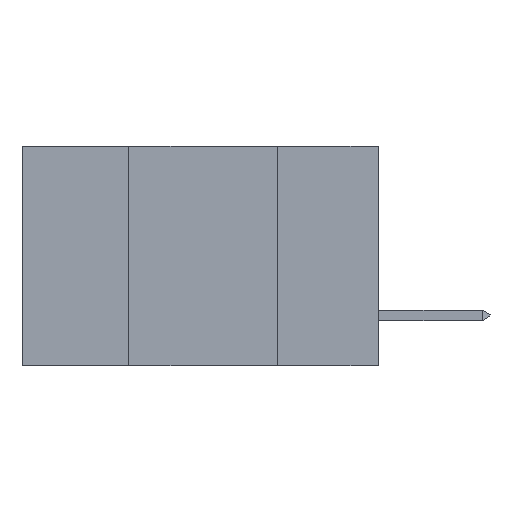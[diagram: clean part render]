
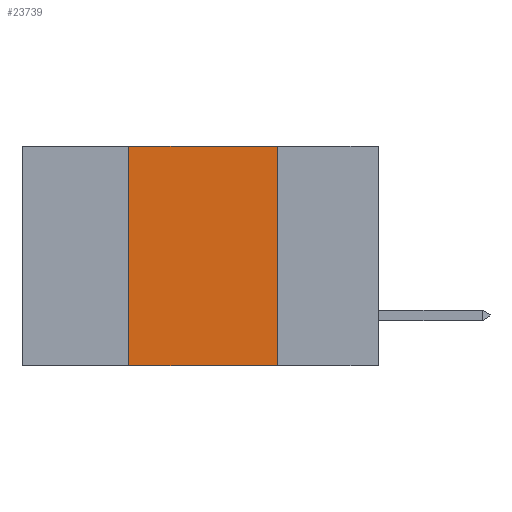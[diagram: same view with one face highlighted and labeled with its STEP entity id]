
A CAD part, left-side view. The second image highlights one B-rep face of the part: STEP entity #23739.
In plain terms, the highlighted planar face has unit normal (-1, 0, 0).
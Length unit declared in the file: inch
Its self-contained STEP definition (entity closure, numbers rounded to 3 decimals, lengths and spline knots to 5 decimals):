
#578 = VERTEX_POINT ( 'NONE', #14400 ) ;
#1663 = VERTEX_POINT ( 'NONE', #5043 ) ;
#1740 = LINE ( 'NONE', #17953, #16033 ) ;
#1945 = CARTESIAN_POINT ( 'NONE',  ( 0., 0.17, -0.37 ) ) ;
#2069 = CARTESIAN_POINT ( 'NONE',  ( 0., 0.6, 0. ) ) ;
#2489 = PLANE ( 'NONE',  #9022 ) ;
#2775 = CARTESIAN_POINT ( 'NONE',  ( 0., 0.17, 0. ) ) ;
#3813 = EDGE_CURVE ( 'NONE', #1663, #17884, #1740, .T. ) ;
#4269 = DIRECTION ( 'NONE',  ( 1., 0., 0. ) ) ;
#4556 = DIRECTION ( 'NONE',  ( 0., 0., -1. ) ) ;
#5043 = CARTESIAN_POINT ( 'NONE',  ( 0., 0.42, 0. ) ) ;
#5257 = LINE ( 'NONE', #8693, #20421 ) ;
#7491 = VECTOR ( 'NONE', #14513, 39.37008 ) ;
#8693 = CARTESIAN_POINT ( 'NONE',  ( 0., 0.42, 0. ) ) ;
#8917 = LINE ( 'NONE', #17741, #9829 ) ;
#8945 = DIRECTION ( 'NONE',  ( 0., 0., 1. ) ) ;
#9022 = AXIS2_PLACEMENT_3D ( 'NONE', #2069, #4269, #9516 ) ;
#9349 = EDGE_CURVE ( 'NONE', #578, #1663, #5257, .T. ) ;
#9516 = DIRECTION ( 'NONE',  ( 0., 0., -1. ) ) ;
#9829 = VECTOR ( 'NONE', #4556, 39.37008 ) ;
#10292 = ORIENTED_EDGE ( 'NONE', *, *, #3813, .F. ) ;
#11657 = EDGE_LOOP ( 'NONE', ( #18509, #10292, #17212, #16828 ) ) ;
#12730 = EDGE_CURVE ( 'NONE', #578, #19247, #23510, .T. ) ;
#13642 = FACE_OUTER_BOUND ( 'NONE', #11657, .T. ) ;
#14400 = CARTESIAN_POINT ( 'NONE',  ( 0., 0.42, -0.37 ) ) ;
#14422 = EDGE_CURVE ( 'NONE', #17884, #19247, #8917, .T. ) ;
#14513 = DIRECTION ( 'NONE',  ( 0., -1., 0. ) ) ;
#16033 = VECTOR ( 'NONE', #16200, 39.37008 ) ;
#16200 = DIRECTION ( 'NONE',  ( 0., -1., 0. ) ) ;
#16828 = ORIENTED_EDGE ( 'NONE', *, *, #12730, .T. ) ;
#17212 = ORIENTED_EDGE ( 'NONE', *, *, #9349, .F. ) ;
#17741 = CARTESIAN_POINT ( 'NONE',  ( 0., 0.17, 0. ) ) ;
#17884 = VERTEX_POINT ( 'NONE', #2775 ) ;
#17953 = CARTESIAN_POINT ( 'NONE',  ( 0., 0.6, 0. ) ) ;
#18509 = ORIENTED_EDGE ( 'NONE', *, *, #14422, .F. ) ;
#19247 = VERTEX_POINT ( 'NONE', #1945 ) ;
#20020 = CARTESIAN_POINT ( 'NONE',  ( 0., 0.6, -0.37 ) ) ;
#20421 = VECTOR ( 'NONE', #8945, 39.37008 ) ;
#23510 = LINE ( 'NONE', #20020, #7491 ) ;
#23739 = ADVANCED_FACE ( 'NONE', ( #13642 ), #2489, .F. ) ;
